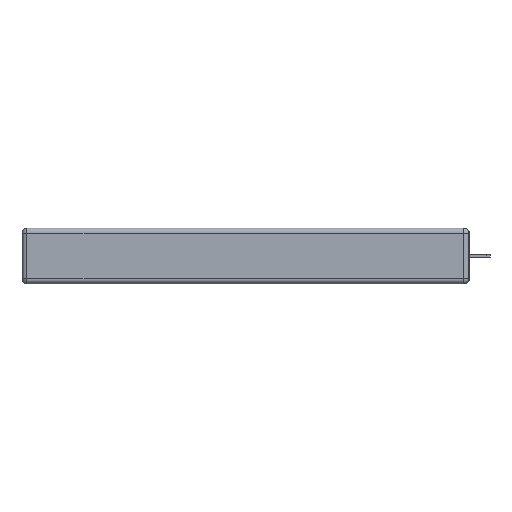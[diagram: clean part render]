
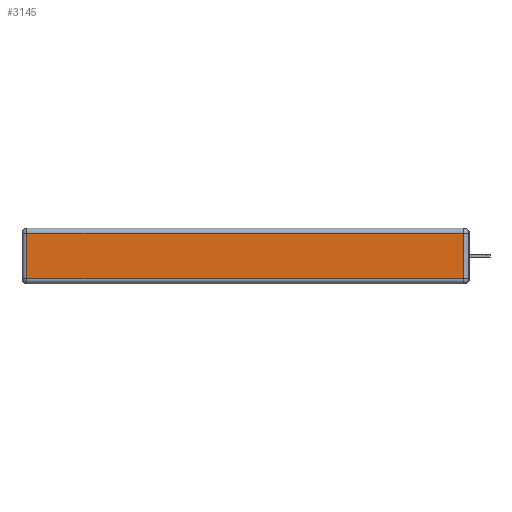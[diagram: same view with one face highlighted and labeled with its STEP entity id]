
A CAD part, left-side view. The second image highlights one B-rep face of the part: STEP entity #3145.
In plain terms, the highlighted planar face has unit normal (-1, 0, 0).
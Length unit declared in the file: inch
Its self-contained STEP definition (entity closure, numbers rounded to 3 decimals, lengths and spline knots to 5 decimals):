
#259 = CARTESIAN_POINT ( 'NONE',  ( 0., 0., -0.313 ) ) ;
#314 = DIRECTION ( 'NONE',  ( 0., 0., 1. ) ) ;
#1349 = FACE_OUTER_BOUND ( 'NONE', #10302, .T. ) ;
#2502 = DIRECTION ( 'NONE',  ( 0., 0., -1. ) ) ;
#2520 = VECTOR ( 'NONE', #2502, 39.37008 ) ;
#2968 = EDGE_CURVE ( 'NONE', #14281, #10472, #5948, .T. ) ;
#3145 = ADVANCED_FACE ( 'NONE', ( #1349 ), #6358, .T. ) ;
#3789 = CARTESIAN_POINT ( 'NONE',  ( 0., 2.72, -0.313 ) ) ;
#3897 = DIRECTION ( 'NONE',  ( -1., 0., 0. ) ) ;
#4815 = CARTESIAN_POINT ( 'NONE',  ( 0., 0.03, -0.03 ) ) ;
#5439 = CARTESIAN_POINT ( 'NONE',  ( 0., 2.75, -0.03 ) ) ;
#5518 = EDGE_CURVE ( 'NONE', #10472, #6957, #10420, .T. ) ;
#5535 = ORIENTED_EDGE ( 'NONE', *, *, #5518, .T. ) ;
#5948 = LINE ( 'NONE', #13730, #2520 ) ;
#6358 = PLANE ( 'NONE',  #9930 ) ;
#6386 = CARTESIAN_POINT ( 'NONE',  ( 0., 2.72, -0.03 ) ) ;
#6664 = DIRECTION ( 'NONE',  ( 0., 1., 0. ) ) ;
#6938 = VECTOR ( 'NONE', #9189, 39.37008 ) ;
#6957 = VERTEX_POINT ( 'NONE', #12587 ) ;
#7673 = ORIENTED_EDGE ( 'NONE', *, *, #2968, .T. ) ;
#7739 = LINE ( 'NONE', #5439, #11737 ) ;
#8030 = CARTESIAN_POINT ( 'NONE',  ( 0., 0.03, -0.343 ) ) ;
#8164 = EDGE_CURVE ( 'NONE', #6957, #9661, #9328, .T. ) ;
#9189 = DIRECTION ( 'NONE',  ( 0., -1., 0. ) ) ;
#9328 = LINE ( 'NONE', #8030, #12247 ) ;
#9661 = VERTEX_POINT ( 'NONE', #4815 ) ;
#9930 = AXIS2_PLACEMENT_3D ( 'NONE', #15129, #3897, #13892 ) ;
#10302 = EDGE_LOOP ( 'NONE', ( #5535, #12708, #14229, #7673 ) ) ;
#10420 = LINE ( 'NONE', #259, #6938 ) ;
#10472 = VERTEX_POINT ( 'NONE', #3789 ) ;
#11737 = VECTOR ( 'NONE', #6664, 39.37008 ) ;
#12247 = VECTOR ( 'NONE', #314, 39.37008 ) ;
#12587 = CARTESIAN_POINT ( 'NONE',  ( 0., 0.03, -0.313 ) ) ;
#12708 = ORIENTED_EDGE ( 'NONE', *, *, #8164, .T. ) ;
#13730 = CARTESIAN_POINT ( 'NONE',  ( 0., 2.72, -0.343 ) ) ;
#13892 = DIRECTION ( 'NONE',  ( 0., 0., 1. ) ) ;
#14229 = ORIENTED_EDGE ( 'NONE', *, *, #15284, .T. ) ;
#14281 = VERTEX_POINT ( 'NONE', #6386 ) ;
#15129 = CARTESIAN_POINT ( 'NONE',  ( 0., 0., -0.343 ) ) ;
#15284 = EDGE_CURVE ( 'NONE', #9661, #14281, #7739, .T. ) ;
